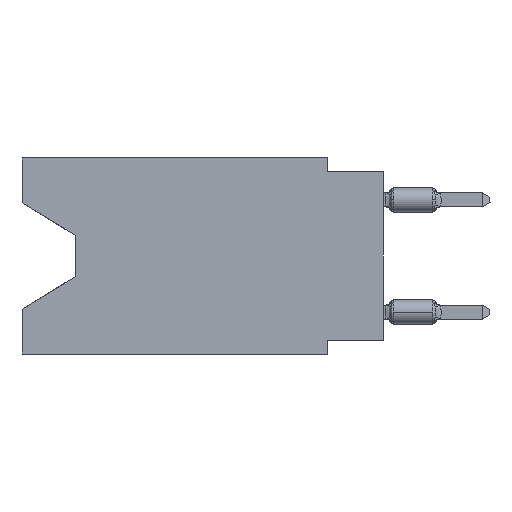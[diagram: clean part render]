
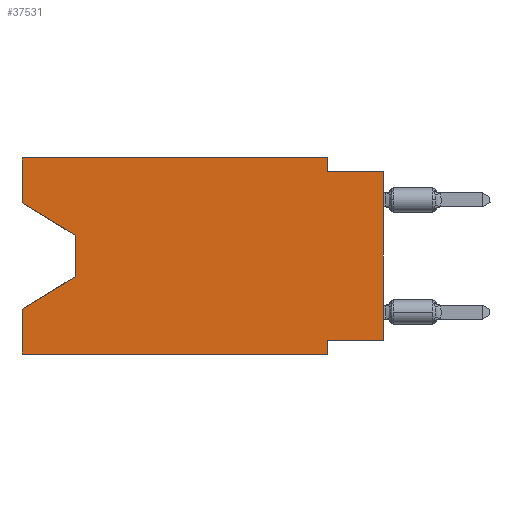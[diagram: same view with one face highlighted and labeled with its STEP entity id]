
A CAD part, left-side view. The second image highlights one B-rep face of the part: STEP entity #37531.
In plain terms, the highlighted planar face has unit normal (-1, 0, 0).
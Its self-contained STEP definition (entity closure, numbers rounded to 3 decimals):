
#364 = VERTEX_POINT ( 'NONE', #1698 ) ;
#464 = CARTESIAN_POINT ( 'NONE',  ( 0., 16.383, 0. ) ) ;
#758 = DIRECTION ( 'NONE',  ( 0., -0.855, -0.519 ) ) ;
#1698 = CARTESIAN_POINT ( 'NONE',  ( 0., 16.383, -8.89 ) ) ;
#2233 = DIRECTION ( 'NONE',  ( 0., 0., 1. ) ) ;
#2735 = DIRECTION ( 'NONE',  ( 0., 0., -1. ) ) ;
#2754 = VERTEX_POINT ( 'NONE', #38142 ) ;
#2962 = EDGE_CURVE ( 'NONE', #42100, #61126, #11418, .T. ) ;
#2977 = VECTOR ( 'NONE', #8717, 1000. ) ;
#3596 = CARTESIAN_POINT ( 'NONE',  ( 0., 2.54, 0. ) ) ;
#4893 = ORIENTED_EDGE ( 'NONE', *, *, #50574, .T. ) ;
#5033 = CARTESIAN_POINT ( 'NONE',  ( 0., 16.383, -2.038 ) ) ;
#6009 = EDGE_CURVE ( 'NONE', #21790, #33623, #39975, .T. ) ;
#6468 = EDGE_CURVE ( 'NONE', #7279, #12307, #17163, .T. ) ;
#7279 = VERTEX_POINT ( 'NONE', #52407 ) ;
#8717 = DIRECTION ( 'NONE',  ( 0., 1., 0. ) ) ;
#10173 = VERTEX_POINT ( 'NONE', #5033 ) ;
#10403 = FACE_OUTER_BOUND ( 'NONE', #21995, .T. ) ;
#11170 = ORIENTED_EDGE ( 'NONE', *, *, #22265, .F. ) ;
#11418 = LINE ( 'NONE', #35013, #26424 ) ;
#12208 = ORIENTED_EDGE ( 'NONE', *, *, #28186, .F. ) ;
#12307 = VERTEX_POINT ( 'NONE', #24409 ) ;
#12314 = CARTESIAN_POINT ( 'NONE',  ( 0., 0., -8.255 ) ) ;
#13521 = DIRECTION ( 'NONE',  ( 0., -1., 0. ) ) ;
#14120 = DIRECTION ( 'NONE',  ( 1., 0., 0. ) ) ;
#14343 = ORIENTED_EDGE ( 'NONE', *, *, #42986, .T. ) ;
#15059 = DIRECTION ( 'NONE',  ( 0., 0., -1. ) ) ;
#15418 = VECTOR ( 'NONE', #758, 1000. ) ;
#17163 = LINE ( 'NONE', #36085, #36667 ) ;
#17253 = LINE ( 'NONE', #55084, #15418 ) ;
#17770 = DIRECTION ( 'NONE',  ( 0., 0., 1. ) ) ;
#20469 = ORIENTED_EDGE ( 'NONE', *, *, #6009, .T. ) ;
#21317 = ORIENTED_EDGE ( 'NONE', *, *, #35265, .T. ) ;
#21624 = DIRECTION ( 'NONE',  ( 0., 0., -1. ) ) ;
#21790 = VERTEX_POINT ( 'NONE', #23936 ) ;
#21995 = EDGE_LOOP ( 'NONE', ( #21317, #20469, #4893, #43899, #14343, #43147, #11170, #35073, #48475, #12208, #43829, #49770 ) ) ;
#22265 = EDGE_CURVE ( 'NONE', #42754, #7279, #36951, .T. ) ;
#23069 = LINE ( 'NONE', #38811, #37832 ) ;
#23335 = CARTESIAN_POINT ( 'NONE',  ( 0., 16.383, 0. ) ) ;
#23936 = CARTESIAN_POINT ( 'NONE',  ( 0., 13.97, -3.505 ) ) ;
#24144 = LINE ( 'NONE', #32840, #29058 ) ;
#24409 = CARTESIAN_POINT ( 'NONE',  ( 0., 2.54, -8.89 ) ) ;
#25960 = LINE ( 'NONE', #3596, #42002 ) ;
#26058 = LINE ( 'NONE', #26365, #47764 ) ;
#26365 = CARTESIAN_POINT ( 'NONE',  ( 0., 13.97, -5.385 ) ) ;
#26424 = VECTOR ( 'NONE', #30366, 1000. ) ;
#26726 = CARTESIAN_POINT ( 'NONE',  ( 0., 0., 0. ) ) ;
#27141 = EDGE_CURVE ( 'NONE', #10173, #51505, #24144, .T. ) ;
#27173 = CARTESIAN_POINT ( 'NONE',  ( 0., 0., -0.635 ) ) ;
#27496 = CARTESIAN_POINT ( 'NONE',  ( 0., 16.383, -8.89 ) ) ;
#27791 = VECTOR ( 'NONE', #13521, 1000. ) ;
#28186 = EDGE_CURVE ( 'NONE', #2754, #42100, #25960, .T. ) ;
#29058 = VECTOR ( 'NONE', #47416, 1000. ) ;
#29695 = VECTOR ( 'NONE', #2735, 1000. ) ;
#30366 = DIRECTION ( 'NONE',  ( 0., -1., 0. ) ) ;
#30485 = LINE ( 'NONE', #26726, #58112 ) ;
#31352 = EDGE_CURVE ( 'NONE', #364, #36345, #42251, .T. ) ;
#32840 = CARTESIAN_POINT ( 'NONE',  ( 0., 16.383, 0. ) ) ;
#33623 = VERTEX_POINT ( 'NONE', #39421 ) ;
#35013 = CARTESIAN_POINT ( 'NONE',  ( 0., 0., -0.635 ) ) ;
#35073 = ORIENTED_EDGE ( 'NONE', *, *, #36450, .T. ) ;
#35265 = EDGE_CURVE ( 'NONE', #10173, #21790, #17253, .T. ) ;
#36085 = CARTESIAN_POINT ( 'NONE',  ( 0., 2.54, -8.89 ) ) ;
#36345 = VERTEX_POINT ( 'NONE', #48795 ) ;
#36450 = EDGE_CURVE ( 'NONE', #42754, #61126, #30485, .T. ) ;
#36667 = VECTOR ( 'NONE', #42574, 1000. ) ;
#36951 = LINE ( 'NONE', #55280, #2977 ) ;
#37531 = ADVANCED_FACE ( 'NONE', ( #10403 ), #42983, .F. ) ;
#37832 = VECTOR ( 'NONE', #48431, 1000. ) ;
#38142 = CARTESIAN_POINT ( 'NONE',  ( 0., 2.54, 0. ) ) ;
#38811 = CARTESIAN_POINT ( 'NONE',  ( 0., 16.383, 0. ) ) ;
#39421 = CARTESIAN_POINT ( 'NONE',  ( 0., 13.97, -5.385 ) ) ;
#39975 = LINE ( 'NONE', #40594, #29695 ) ;
#40594 = CARTESIAN_POINT ( 'NONE',  ( 0., 13.97, -3.505 ) ) ;
#41384 = CARTESIAN_POINT ( 'NONE',  ( 0., 16.383, 0. ) ) ;
#42002 = VECTOR ( 'NONE', #21624, 1000. ) ;
#42100 = VERTEX_POINT ( 'NONE', #43762 ) ;
#42251 = LINE ( 'NONE', #23335, #57179 ) ;
#42385 = AXIS2_PLACEMENT_3D ( 'NONE', #464, #14120, #15059 ) ;
#42574 = DIRECTION ( 'NONE',  ( 0., 0., -1. ) ) ;
#42754 = VERTEX_POINT ( 'NONE', #12314 ) ;
#42983 = PLANE ( 'NONE',  #42385 ) ;
#42986 = EDGE_CURVE ( 'NONE', #364, #12307, #47355, .T. ) ;
#43147 = ORIENTED_EDGE ( 'NONE', *, *, #6468, .F. ) ;
#43762 = CARTESIAN_POINT ( 'NONE',  ( 0., 2.54, -0.635 ) ) ;
#43829 = ORIENTED_EDGE ( 'NONE', *, *, #50466, .F. ) ;
#43899 = ORIENTED_EDGE ( 'NONE', *, *, #31352, .F. ) ;
#47355 = LINE ( 'NONE', #27496, #27791 ) ;
#47416 = DIRECTION ( 'NONE',  ( 0., 0., 1. ) ) ;
#47764 = VECTOR ( 'NONE', #53700, 1000. ) ;
#48431 = DIRECTION ( 'NONE',  ( 0., -1., 0. ) ) ;
#48475 = ORIENTED_EDGE ( 'NONE', *, *, #2962, .F. ) ;
#48795 = CARTESIAN_POINT ( 'NONE',  ( 0., 16.383, -6.852 ) ) ;
#49770 = ORIENTED_EDGE ( 'NONE', *, *, #27141, .F. ) ;
#50466 = EDGE_CURVE ( 'NONE', #51505, #2754, #23069, .T. ) ;
#50574 = EDGE_CURVE ( 'NONE', #33623, #36345, #26058, .T. ) ;
#51505 = VERTEX_POINT ( 'NONE', #41384 ) ;
#52407 = CARTESIAN_POINT ( 'NONE',  ( 0., 2.54, -8.255 ) ) ;
#53700 = DIRECTION ( 'NONE',  ( 0., 0.855, -0.519 ) ) ;
#55084 = CARTESIAN_POINT ( 'NONE',  ( 0., 16.383, -2.038 ) ) ;
#55280 = CARTESIAN_POINT ( 'NONE',  ( 0., 0., -8.255 ) ) ;
#57179 = VECTOR ( 'NONE', #17770, 1000. ) ;
#58112 = VECTOR ( 'NONE', #2233, 1000. ) ;
#61126 = VERTEX_POINT ( 'NONE', #27173 ) ;
